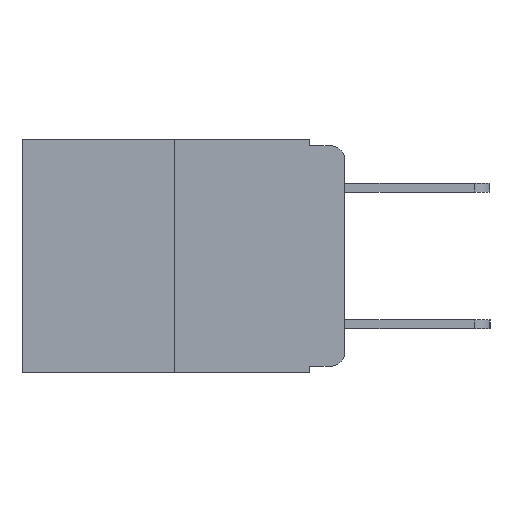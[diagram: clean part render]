
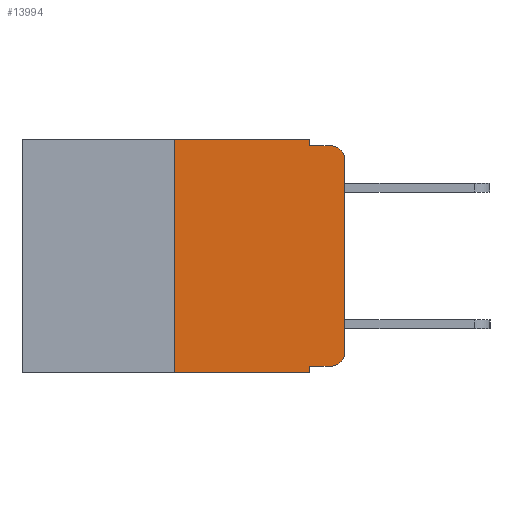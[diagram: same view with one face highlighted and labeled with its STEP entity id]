
A CAD part, left-side view. The second image highlights one B-rep face of the part: STEP entity #13994.
In plain terms, the highlighted planar face has unit normal (-1, 0, 0).
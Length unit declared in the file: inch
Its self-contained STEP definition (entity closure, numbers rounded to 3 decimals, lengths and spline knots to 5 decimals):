
#481 = ORIENTED_EDGE ( 'NONE', *, *, #7777, .F. ) ;
#588 = CARTESIAN_POINT ( 'NONE',  ( 0., 0.02, -0.01 ) ) ;
#604 = FACE_OUTER_BOUND ( 'NONE', #13121, .T. ) ;
#692 = VECTOR ( 'NONE', #13623, 39.37008 ) ;
#737 = LINE ( 'NONE', #12709, #11765 ) ;
#880 = ORIENTED_EDGE ( 'NONE', *, *, #7422, .T. ) ;
#893 = ORIENTED_EDGE ( 'NONE', *, *, #3095, .T. ) ;
#931 = CARTESIAN_POINT ( 'NONE',  ( 0., 0., -0.313 ) ) ;
#981 = LINE ( 'NONE', #8627, #1747 ) ;
#1162 = VERTEX_POINT ( 'NONE', #588 ) ;
#1610 = DIRECTION ( 'NONE',  ( 0., 0., -1. ) ) ;
#1698 = CARTESIAN_POINT ( 'NONE',  ( 0., 0.02, -0.313 ) ) ;
#1747 = VECTOR ( 'NONE', #5459, 39.37008 ) ;
#2139 = VERTEX_POINT ( 'NONE', #7356 ) ;
#2285 = DIRECTION ( 'NONE',  ( 0., -1., 0. ) ) ;
#2355 = VERTEX_POINT ( 'NONE', #7124 ) ;
#2553 = VERTEX_POINT ( 'NONE', #2958 ) ;
#2711 = CARTESIAN_POINT ( 'NONE',  ( 0., 0.051, -0.01 ) ) ;
#2750 = EDGE_CURVE ( 'NONE', #8466, #4661, #12489, .T. ) ;
#2802 = CIRCLE ( 'NONE', #6875, 0.02 ) ;
#2958 = CARTESIAN_POINT ( 'NONE',  ( 0., 0.25, 0. ) ) ;
#2968 = CARTESIAN_POINT ( 'NONE',  ( 0., 0.02, -0.03 ) ) ;
#3095 = EDGE_CURVE ( 'NONE', #6915, #2139, #3469, .T. ) ;
#3469 = LINE ( 'NONE', #5608, #7744 ) ;
#3952 = EDGE_CURVE ( 'NONE', #7126, #2355, #9752, .T. ) ;
#4040 = CARTESIAN_POINT ( 'NONE',  ( 0., 0., -0.03 ) ) ;
#4582 = VECTOR ( 'NONE', #1610, 39.37008 ) ;
#4610 = CARTESIAN_POINT ( 'NONE',  ( 0., 0.25, -0.343 ) ) ;
#4646 = CARTESIAN_POINT ( 'NONE',  ( 0., 0.473, -0.343 ) ) ;
#4661 = VERTEX_POINT ( 'NONE', #4040 ) ;
#5065 = DIRECTION ( 'NONE',  ( 1., 0., 0. ) ) ;
#5161 = DIRECTION ( 'NONE',  ( -1., 0., 0. ) ) ;
#5178 = ORIENTED_EDGE ( 'NONE', *, *, #8314, .F. ) ;
#5261 = ORIENTED_EDGE ( 'NONE', *, *, #2750, .T. ) ;
#5283 = VECTOR ( 'NONE', #7456, 39.37008 ) ;
#5327 = ORIENTED_EDGE ( 'NONE', *, *, #3952, .T. ) ;
#5403 = LINE ( 'NONE', #12048, #5283 ) ;
#5459 = DIRECTION ( 'NONE',  ( 0., -1., 0. ) ) ;
#5608 = CARTESIAN_POINT ( 'NONE',  ( 0., 0.051, -0.333 ) ) ;
#5826 = EDGE_CURVE ( 'NONE', #13987, #7339, #12237, .T. ) ;
#6011 = DIRECTION ( 'NONE',  ( -1., 0., 0. ) ) ;
#6268 = DIRECTION ( 'NONE',  ( 0., 0., -1. ) ) ;
#6280 = AXIS2_PLACEMENT_3D ( 'NONE', #12576, #5065, #13504 ) ;
#6599 = AXIS2_PLACEMENT_3D ( 'NONE', #1698, #6011, #13607 ) ;
#6875 = AXIS2_PLACEMENT_3D ( 'NONE', #2968, #5161, #8619 ) ;
#6915 = VERTEX_POINT ( 'NONE', #10427 ) ;
#6993 = CARTESIAN_POINT ( 'NONE',  ( 0., 0.051, 0. ) ) ;
#7036 = CARTESIAN_POINT ( 'NONE',  ( 0., 0., 0. ) ) ;
#7124 = CARTESIAN_POINT ( 'NONE',  ( 0., 0.051, -0.343 ) ) ;
#7126 = VERTEX_POINT ( 'NONE', #4610 ) ;
#7240 = ORIENTED_EDGE ( 'NONE', *, *, #12739, .F. ) ;
#7339 = VERTEX_POINT ( 'NONE', #2711 ) ;
#7356 = CARTESIAN_POINT ( 'NONE',  ( 0., 0.02, -0.333 ) ) ;
#7422 = EDGE_CURVE ( 'NONE', #2139, #8466, #10883, .T. ) ;
#7456 = DIRECTION ( 'NONE',  ( 0., -1., 0. ) ) ;
#7744 = VECTOR ( 'NONE', #2285, 39.37008 ) ;
#7777 = EDGE_CURVE ( 'NONE', #7126, #2553, #737, .T. ) ;
#7825 = DIRECTION ( 'NONE',  ( 0., -1., 0. ) ) ;
#8159 = ORIENTED_EDGE ( 'NONE', *, *, #13179, .F. ) ;
#8288 = VECTOR ( 'NONE', #7825, 39.37008 ) ;
#8314 = EDGE_CURVE ( 'NONE', #7339, #1162, #5403, .T. ) ;
#8466 = VERTEX_POINT ( 'NONE', #931 ) ;
#8619 = DIRECTION ( 'NONE',  ( 0., 0., -1. ) ) ;
#8627 = CARTESIAN_POINT ( 'NONE',  ( 0., 0.473, 0. ) ) ;
#9752 = LINE ( 'NONE', #4646, #8288 ) ;
#9926 = ORIENTED_EDGE ( 'NONE', *, *, #5826, .F. ) ;
#10427 = CARTESIAN_POINT ( 'NONE',  ( 0., 0.051, -0.333 ) ) ;
#10519 = CARTESIAN_POINT ( 'NONE',  ( 0., 0.051, 0. ) ) ;
#10537 = EDGE_CURVE ( 'NONE', #4661, #1162, #2802, .T. ) ;
#10540 = VECTOR ( 'NONE', #6268, 39.37008 ) ;
#10883 = CIRCLE ( 'NONE', #6599, 0.02 ) ;
#11096 = ORIENTED_EDGE ( 'NONE', *, *, #10537, .T. ) ;
#11303 = PLANE ( 'NONE',  #6280 ) ;
#11501 = CARTESIAN_POINT ( 'NONE',  ( 0., 0.051, 0. ) ) ;
#11765 = VECTOR ( 'NONE', #13845, 39.37008 ) ;
#12048 = CARTESIAN_POINT ( 'NONE',  ( 0., 0.051, -0.01 ) ) ;
#12237 = LINE ( 'NONE', #6993, #4582 ) ;
#12489 = LINE ( 'NONE', #7036, #692 ) ;
#12576 = CARTESIAN_POINT ( 'NONE',  ( 0., 0.473, 0. ) ) ;
#12709 = CARTESIAN_POINT ( 'NONE',  ( 0., 0.25, 0. ) ) ;
#12739 = EDGE_CURVE ( 'NONE', #6915, #2355, #13710, .T. ) ;
#13121 = EDGE_LOOP ( 'NONE', ( #5261, #11096, #5178, #9926, #8159, #481, #5327, #7240, #893, #880 ) ) ;
#13179 = EDGE_CURVE ( 'NONE', #2553, #13987, #981, .T. ) ;
#13504 = DIRECTION ( 'NONE',  ( 0., 0., -1. ) ) ;
#13607 = DIRECTION ( 'NONE',  ( 0., 0., -1. ) ) ;
#13623 = DIRECTION ( 'NONE',  ( 0., 0., 1. ) ) ;
#13710 = LINE ( 'NONE', #11501, #10540 ) ;
#13845 = DIRECTION ( 'NONE',  ( 0., 0., 1. ) ) ;
#13987 = VERTEX_POINT ( 'NONE', #10519 ) ;
#13994 = ADVANCED_FACE ( 'NONE', ( #604 ), #11303, .F. ) ;
